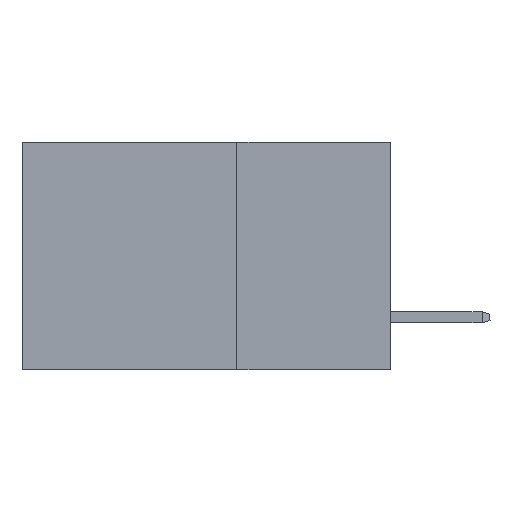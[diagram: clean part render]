
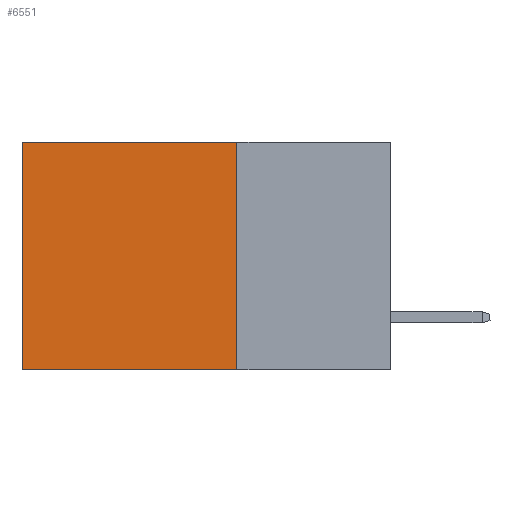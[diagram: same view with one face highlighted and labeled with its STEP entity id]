
A CAD part, left-side view. The second image highlights one B-rep face of the part: STEP entity #6551.
In plain terms, the highlighted planar face has unit normal (-1, 0, 0).
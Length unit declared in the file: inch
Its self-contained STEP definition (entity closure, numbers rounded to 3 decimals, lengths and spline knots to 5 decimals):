
#363 = FACE_OUTER_BOUND ( 'NONE', #2606, .T. ) ;
#1411 = VECTOR ( 'NONE', #11435, 39.37008 ) ;
#1796 = LINE ( 'NONE', #13119, #13146 ) ;
#1831 = VERTEX_POINT ( 'NONE', #5942 ) ;
#2284 = DIRECTION ( 'NONE',  ( 1., 0., 0. ) ) ;
#2606 = EDGE_LOOP ( 'NONE', ( #11223, #11213, #11929, #2959 ) ) ;
#2657 = VERTEX_POINT ( 'NONE', #6686 ) ;
#2883 = LINE ( 'NONE', #6838, #11340 ) ;
#2959 = ORIENTED_EDGE ( 'NONE', *, *, #9382, .T. ) ;
#3346 = CARTESIAN_POINT ( 'NONE',  ( 0.2875, 0.25, 0. ) ) ;
#4489 = LINE ( 'NONE', #3346, #9923 ) ;
#5651 = DIRECTION ( 'NONE',  ( 0., 0., -1. ) ) ;
#5723 = CARTESIAN_POINT ( 'NONE',  ( 0.2875, 0.25, 0. ) ) ;
#5942 = CARTESIAN_POINT ( 'NONE',  ( 0.2875, 0.25, 0. ) ) ;
#6551 = ADVANCED_FACE ( 'NONE', ( #363 ), #8960, .F. ) ;
#6686 = CARTESIAN_POINT ( 'NONE',  ( 0.2875, 0.6, -0.37 ) ) ;
#6838 = CARTESIAN_POINT ( 'NONE',  ( 0.2875, 0.25, -0.37 ) ) ;
#6873 = VERTEX_POINT ( 'NONE', #9494 ) ;
#7686 = CARTESIAN_POINT ( 'NONE',  ( 0.2875, 0.25, -0.37 ) ) ;
#8506 = EDGE_CURVE ( 'NONE', #6873, #2657, #1796, .T. ) ;
#8960 = PLANE ( 'NONE',  #13337 ) ;
#9382 = EDGE_CURVE ( 'NONE', #1831, #6873, #13118, .T. ) ;
#9494 = CARTESIAN_POINT ( 'NONE',  ( 0.2875, 0.6, 0. ) ) ;
#9739 = EDGE_CURVE ( 'NONE', #13870, #2657, #2883, .T. ) ;
#9923 = VECTOR ( 'NONE', #12100, 39.37008 ) ;
#10049 = DIRECTION ( 'NONE',  ( 0., 0., -1. ) ) ;
#10340 = CARTESIAN_POINT ( 'NONE',  ( 0.2875, 0.25, 0. ) ) ;
#11213 = ORIENTED_EDGE ( 'NONE', *, *, #9739, .F. ) ;
#11223 = ORIENTED_EDGE ( 'NONE', *, *, #8506, .T. ) ;
#11340 = VECTOR ( 'NONE', #14287, 39.37008 ) ;
#11435 = DIRECTION ( 'NONE',  ( 0., 1., 0. ) ) ;
#11929 = ORIENTED_EDGE ( 'NONE', *, *, #13312, .F. ) ;
#12100 = DIRECTION ( 'NONE',  ( 0., 0., -1. ) ) ;
#13118 = LINE ( 'NONE', #10340, #1411 ) ;
#13119 = CARTESIAN_POINT ( 'NONE',  ( 0.2875, 0.6, 0. ) ) ;
#13146 = VECTOR ( 'NONE', #5651, 39.37008 ) ;
#13312 = EDGE_CURVE ( 'NONE', #1831, #13870, #4489, .T. ) ;
#13337 = AXIS2_PLACEMENT_3D ( 'NONE', #5723, #2284, #10049 ) ;
#13870 = VERTEX_POINT ( 'NONE', #7686 ) ;
#14287 = DIRECTION ( 'NONE',  ( 0., 1., 0. ) ) ;
